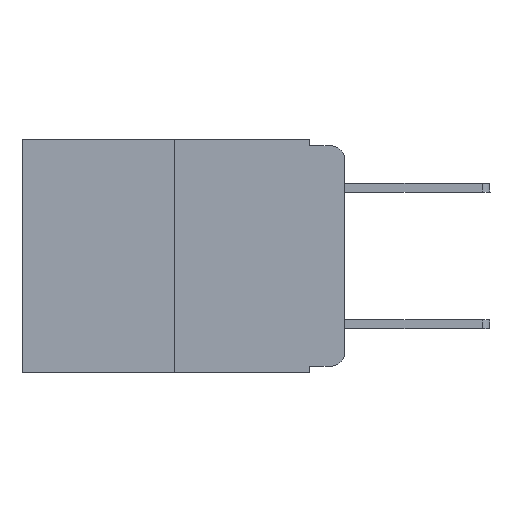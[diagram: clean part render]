
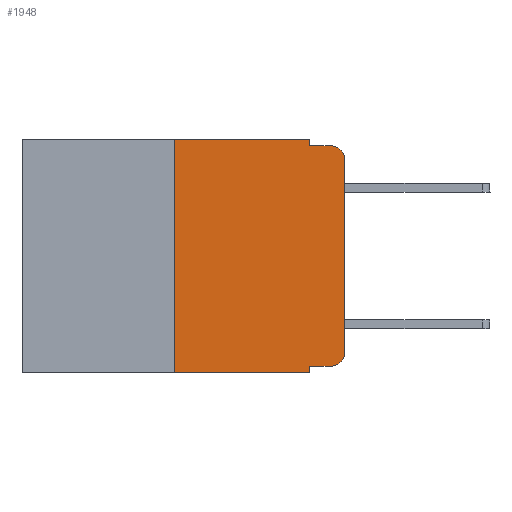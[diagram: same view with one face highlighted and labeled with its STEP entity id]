
A CAD part, left-side view. The second image highlights one B-rep face of the part: STEP entity #1948.
In plain terms, the highlighted planar face has unit normal (-1, 0, 0).
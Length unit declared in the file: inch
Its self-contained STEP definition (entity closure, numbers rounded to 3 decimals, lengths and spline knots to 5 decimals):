
#637 = EDGE_CURVE ( 'NONE', #15463, #10090, #10161, .T. ) ;
#1255 = EDGE_CURVE ( 'NONE', #2628, #15463, #3698, .T. ) ;
#1264 = CARTESIAN_POINT ( 'NONE',  ( 0., 0.473, 0. ) ) ;
#1485 = VERTEX_POINT ( 'NONE', #2823 ) ;
#1525 = AXIS2_PLACEMENT_3D ( 'NONE', #7944, #18226, #3670 ) ;
#1737 = VERTEX_POINT ( 'NONE', #7074 ) ;
#1843 = EDGE_CURVE ( 'NONE', #4263, #1737, #2331, .T. ) ;
#1948 = ADVANCED_FACE ( 'NONE', ( #15350 ), #18713, .F. ) ;
#2025 = CARTESIAN_POINT ( 'NONE',  ( 0., 0.473, -0.343 ) ) ;
#2096 = ORIENTED_EDGE ( 'NONE', *, *, #1843, .T. ) ;
#2331 = LINE ( 'NONE', #12382, #9571 ) ;
#2513 = CARTESIAN_POINT ( 'NONE',  ( 0., 0., 0. ) ) ;
#2628 = VERTEX_POINT ( 'NONE', #18003 ) ;
#2823 = CARTESIAN_POINT ( 'NONE',  ( 0., 0., -0.03 ) ) ;
#3620 = VECTOR ( 'NONE', #5972, 39.37008 ) ;
#3670 = DIRECTION ( 'NONE',  ( 0., 0., -1. ) ) ;
#3698 = LINE ( 'NONE', #12582, #16132 ) ;
#3873 = DIRECTION ( 'NONE',  ( 0., -1., 0. ) ) ;
#4043 = VECTOR ( 'NONE', #13290, 39.37008 ) ;
#4263 = VERTEX_POINT ( 'NONE', #11753 ) ;
#4432 = DIRECTION ( 'NONE',  ( 0., -1., 0. ) ) ;
#4557 = LINE ( 'NONE', #10381, #3620 ) ;
#4882 = ORIENTED_EDGE ( 'NONE', *, *, #15209, .T. ) ;
#5026 = CARTESIAN_POINT ( 'NONE',  ( 0., 0.051, -0.01 ) ) ;
#5134 = VERTEX_POINT ( 'NONE', #8640 ) ;
#5490 = CIRCLE ( 'NONE', #8547, 0.02 ) ;
#5972 = DIRECTION ( 'NONE',  ( 0., 0., -1. ) ) ;
#6089 = ORIENTED_EDGE ( 'NONE', *, *, #12216, .T. ) ;
#6497 = CARTESIAN_POINT ( 'NONE',  ( 0., 0.25, 0. ) ) ;
#6891 = AXIS2_PLACEMENT_3D ( 'NONE', #1264, #12952, #8537 ) ;
#7074 = CARTESIAN_POINT ( 'NONE',  ( 0., 0.02, -0.333 ) ) ;
#7207 = ORIENTED_EDGE ( 'NONE', *, *, #1255, .F. ) ;
#7253 = EDGE_LOOP ( 'NONE', ( #4882, #6089, #13719, #13815, #16698, #7207, #14771, #7524, #2096, #15103 ) ) ;
#7369 = VECTOR ( 'NONE', #11318, 39.37008 ) ;
#7446 = LINE ( 'NONE', #8978, #4043 ) ;
#7524 = ORIENTED_EDGE ( 'NONE', *, *, #10460, .F. ) ;
#7944 = CARTESIAN_POINT ( 'NONE',  ( 0., 0.02, -0.313 ) ) ;
#8434 = LINE ( 'NONE', #2513, #7369 ) ;
#8537 = DIRECTION ( 'NONE',  ( 0., 0., -1. ) ) ;
#8547 = AXIS2_PLACEMENT_3D ( 'NONE', #14780, #17938, #13617 ) ;
#8640 = CARTESIAN_POINT ( 'NONE',  ( 0., 0., -0.313 ) ) ;
#8746 = VECTOR ( 'NONE', #4432, 39.37008 ) ;
#8978 = CARTESIAN_POINT ( 'NONE',  ( 0., 0.051, 0. ) ) ;
#9571 = VECTOR ( 'NONE', #3873, 39.37008 ) ;
#10090 = VERTEX_POINT ( 'NONE', #16840 ) ;
#10161 = LINE ( 'NONE', #13403, #8746 ) ;
#10361 = DIRECTION ( 'NONE',  ( 0., -1., 0. ) ) ;
#10381 = CARTESIAN_POINT ( 'NONE',  ( 0., 0.051, 0. ) ) ;
#10460 = EDGE_CURVE ( 'NONE', #4263, #18216, #4557, .T. ) ;
#10739 = LINE ( 'NONE', #2025, #10991 ) ;
#10991 = VECTOR ( 'NONE', #10361, 39.37008 ) ;
#11318 = DIRECTION ( 'NONE',  ( 0., 0., 1. ) ) ;
#11753 = CARTESIAN_POINT ( 'NONE',  ( 0., 0.051, -0.333 ) ) ;
#11803 = VERTEX_POINT ( 'NONE', #5026 ) ;
#12216 = EDGE_CURVE ( 'NONE', #1485, #13165, #5490, .T. ) ;
#12330 = EDGE_CURVE ( 'NONE', #2628, #18216, #10739, .T. ) ;
#12382 = CARTESIAN_POINT ( 'NONE',  ( 0., 0.051, -0.333 ) ) ;
#12522 = EDGE_CURVE ( 'NONE', #1737, #5134, #13154, .T. ) ;
#12582 = CARTESIAN_POINT ( 'NONE',  ( 0., 0.25, 0. ) ) ;
#12610 = VECTOR ( 'NONE', #18524, 39.37008 ) ;
#12819 = CARTESIAN_POINT ( 'NONE',  ( 0., 0.02, -0.01 ) ) ;
#12932 = CARTESIAN_POINT ( 'NONE',  ( 0., 0.051, -0.343 ) ) ;
#12952 = DIRECTION ( 'NONE',  ( 1., 0., 0. ) ) ;
#13154 = CIRCLE ( 'NONE', #1525, 0.02 ) ;
#13165 = VERTEX_POINT ( 'NONE', #12819 ) ;
#13290 = DIRECTION ( 'NONE',  ( 0., 0., -1. ) ) ;
#13403 = CARTESIAN_POINT ( 'NONE',  ( 0., 0.473, 0. ) ) ;
#13617 = DIRECTION ( 'NONE',  ( 0., 0., -1. ) ) ;
#13719 = ORIENTED_EDGE ( 'NONE', *, *, #16495, .F. ) ;
#13815 = ORIENTED_EDGE ( 'NONE', *, *, #15800, .F. ) ;
#14201 = LINE ( 'NONE', #15833, #12610 ) ;
#14771 = ORIENTED_EDGE ( 'NONE', *, *, #12330, .T. ) ;
#14780 = CARTESIAN_POINT ( 'NONE',  ( 0., 0.02, -0.03 ) ) ;
#15103 = ORIENTED_EDGE ( 'NONE', *, *, #12522, .T. ) ;
#15209 = EDGE_CURVE ( 'NONE', #5134, #1485, #8434, .T. ) ;
#15350 = FACE_OUTER_BOUND ( 'NONE', #7253, .T. ) ;
#15463 = VERTEX_POINT ( 'NONE', #6497 ) ;
#15800 = EDGE_CURVE ( 'NONE', #10090, #11803, #7446, .T. ) ;
#15833 = CARTESIAN_POINT ( 'NONE',  ( 0., 0.051, -0.01 ) ) ;
#16132 = VECTOR ( 'NONE', #18345, 39.37008 ) ;
#16495 = EDGE_CURVE ( 'NONE', #11803, #13165, #14201, .T. ) ;
#16698 = ORIENTED_EDGE ( 'NONE', *, *, #637, .F. ) ;
#16840 = CARTESIAN_POINT ( 'NONE',  ( 0., 0.051, 0. ) ) ;
#17938 = DIRECTION ( 'NONE',  ( -1., 0., 0. ) ) ;
#18003 = CARTESIAN_POINT ( 'NONE',  ( 0., 0.25, -0.343 ) ) ;
#18216 = VERTEX_POINT ( 'NONE', #12932 ) ;
#18226 = DIRECTION ( 'NONE',  ( -1., 0., 0. ) ) ;
#18345 = DIRECTION ( 'NONE',  ( 0., 0., 1. ) ) ;
#18524 = DIRECTION ( 'NONE',  ( 0., -1., 0. ) ) ;
#18713 = PLANE ( 'NONE',  #6891 ) ;
